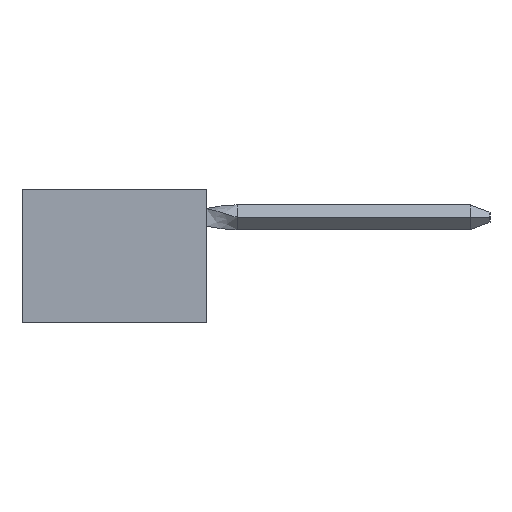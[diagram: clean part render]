
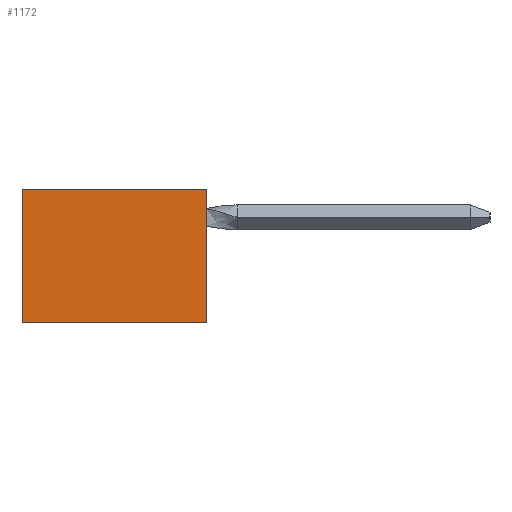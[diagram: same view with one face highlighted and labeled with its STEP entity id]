
A CAD part, left-side view. The second image highlights one B-rep face of the part: STEP entity #1172.
In plain terms, the highlighted planar face has unit normal (-1, 0, 0).
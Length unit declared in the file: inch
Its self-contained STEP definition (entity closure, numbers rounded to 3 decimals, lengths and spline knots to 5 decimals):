
#795 = VECTOR ( 'NONE', #7310, 39.37008 ) ;
#807 = ORIENTED_EDGE ( 'NONE', *, *, #15073, .T. ) ;
#1096 = EDGE_CURVE ( 'NONE', #3323, #18815, #11364, .T. ) ;
#1172 = ADVANCED_FACE ( 'NONE', ( #9744 ), #11894, .F. ) ;
#1326 = LINE ( 'NONE', #19118, #795 ) ;
#3110 = DIRECTION ( 'NONE',  ( 0., 1., 0. ) ) ;
#3193 = DIRECTION ( 'NONE',  ( 0., 0., -1. ) ) ;
#3323 = VERTEX_POINT ( 'NONE', #8000 ) ;
#4619 = VECTOR ( 'NONE', #3110, 39.37008 ) ;
#6488 = CARTESIAN_POINT ( 'NONE',  ( 0.298, -0.027, 0. ) ) ;
#7310 = DIRECTION ( 'NONE',  ( 0., 1., 0. ) ) ;
#7385 = CARTESIAN_POINT ( 'NONE',  ( 0.298, 0., -0.343 ) ) ;
#8000 = CARTESIAN_POINT ( 'NONE',  ( 0.298, 0., 0. ) ) ;
#9744 = FACE_OUTER_BOUND ( 'NONE', #22095, .T. ) ;
#11364 = LINE ( 'NONE', #6488, #4619 ) ;
#11745 = CARTESIAN_POINT ( 'NONE',  ( 0.298, -0.027, 0. ) ) ;
#11828 = DIRECTION ( 'NONE',  ( 0., 0., -1. ) ) ;
#11894 = PLANE ( 'NONE',  #22174 ) ;
#11971 = CARTESIAN_POINT ( 'NONE',  ( 0.298, 0.473, -0.343 ) ) ;
#12092 = LINE ( 'NONE', #21690, #18581 ) ;
#12506 = LINE ( 'NONE', #13493, #17663 ) ;
#13493 = CARTESIAN_POINT ( 'NONE',  ( 0.298, 0.473, 0. ) ) ;
#13647 = CARTESIAN_POINT ( 'NONE',  ( 0.298, 0.473, 0. ) ) ;
#15073 = EDGE_CURVE ( 'NONE', #15579, #3323, #12092, .T. ) ;
#15360 = DIRECTION ( 'NONE',  ( 1., 0., 0. ) ) ;
#15468 = EDGE_CURVE ( 'NONE', #15579, #20865, #1326, .T. ) ;
#15518 = ORIENTED_EDGE ( 'NONE', *, *, #1096, .T. ) ;
#15579 = VERTEX_POINT ( 'NONE', #7385 ) ;
#15629 = ORIENTED_EDGE ( 'NONE', *, *, #15468, .F. ) ;
#17134 = EDGE_CURVE ( 'NONE', #18815, #20865, #12506, .T. ) ;
#17663 = VECTOR ( 'NONE', #3193, 39.37008 ) ;
#18581 = VECTOR ( 'NONE', #19882, 39.37008 ) ;
#18815 = VERTEX_POINT ( 'NONE', #13647 ) ;
#19118 = CARTESIAN_POINT ( 'NONE',  ( 0.298, 0.473, -0.343 ) ) ;
#19882 = DIRECTION ( 'NONE',  ( 0., 0., 1. ) ) ;
#20865 = VERTEX_POINT ( 'NONE', #11971 ) ;
#21527 = ORIENTED_EDGE ( 'NONE', *, *, #17134, .T. ) ;
#21690 = CARTESIAN_POINT ( 'NONE',  ( 0.298, 0., -0.343 ) ) ;
#22095 = EDGE_LOOP ( 'NONE', ( #807, #15518, #21527, #15629 ) ) ;
#22174 = AXIS2_PLACEMENT_3D ( 'NONE', #11745, #15360, #11828 ) ;
